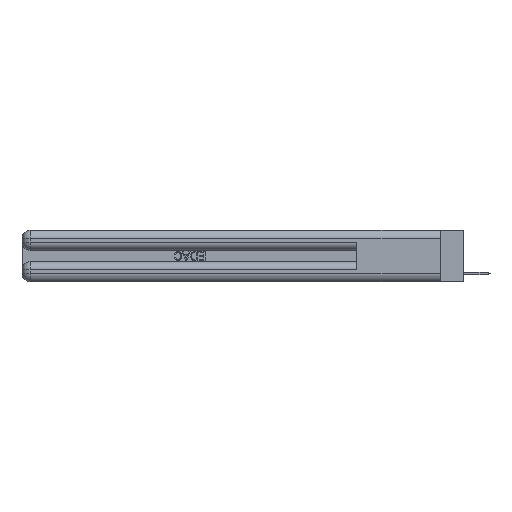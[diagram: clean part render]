
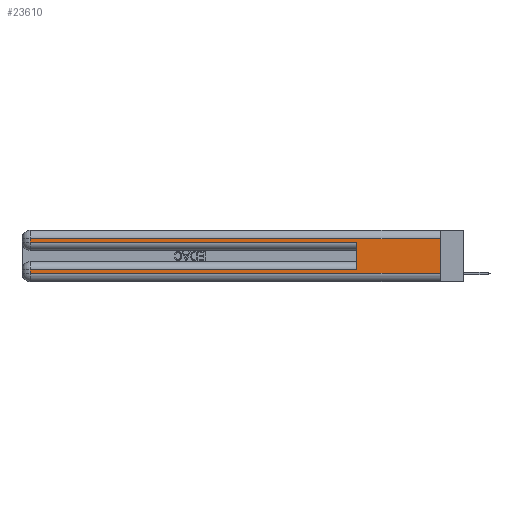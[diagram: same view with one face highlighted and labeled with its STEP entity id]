
A CAD part, left-side view. The second image highlights one B-rep face of the part: STEP entity #23610.
In plain terms, the highlighted planar face has unit normal (-1, 0, 0).
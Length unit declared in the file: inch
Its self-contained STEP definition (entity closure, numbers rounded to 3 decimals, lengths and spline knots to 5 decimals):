
#641 = CARTESIAN_POINT ( 'NONE',  ( 0., 2.94, 0.06 ) ) ;
#1298 = DIRECTION ( 'NONE',  ( 0., 1., 0. ) ) ;
#1534 = ORIENTED_EDGE ( 'NONE', *, *, #5036, .F. ) ;
#1931 = VERTEX_POINT ( 'NONE', #29692 ) ;
#2339 = VERTEX_POINT ( 'NONE', #19806 ) ;
#2497 = VERTEX_POINT ( 'NONE', #4908 ) ;
#2538 = DIRECTION ( 'NONE',  ( 0., 0., -1. ) ) ;
#2982 = DIRECTION ( 'NONE',  ( 0., 0., 1. ) ) ;
#3294 = ORIENTED_EDGE ( 'NONE', *, *, #14458, .T. ) ;
#3583 = DIRECTION ( 'NONE',  ( 0., 0., -1. ) ) ;
#4908 = CARTESIAN_POINT ( 'NONE',  ( 0., 2.94, 0.085 ) ) ;
#4956 = CARTESIAN_POINT ( 'NONE',  ( 0., 0.6, 0.145 ) ) ;
#5036 = EDGE_CURVE ( 'NONE', #18062, #2339, #28475, .T. ) ;
#5630 = VECTOR ( 'NONE', #28234, 39.37008 ) ;
#5827 = EDGE_CURVE ( 'NONE', #1931, #2339, #6057, .T. ) ;
#6057 = LINE ( 'NONE', #8047, #24144 ) ;
#6139 = LINE ( 'NONE', #10268, #23986 ) ;
#6505 = ORIENTED_EDGE ( 'NONE', *, *, #22108, .T. ) ;
#6848 = VECTOR ( 'NONE', #14466, 39.37008 ) ;
#7990 = EDGE_CURVE ( 'NONE', #18062, #2497, #6139, .T. ) ;
#8047 = CARTESIAN_POINT ( 'NONE',  ( 0., 0., 0.285 ) ) ;
#8107 = CARTESIAN_POINT ( 'NONE',  ( 0., 0., 0.06 ) ) ;
#8311 = EDGE_LOOP ( 'NONE', ( #23477, #3294, #29740, #26399, #1534, #8795, #27456, #6505 ) ) ;
#8795 = ORIENTED_EDGE ( 'NONE', *, *, #7990, .T. ) ;
#8894 = EDGE_CURVE ( 'NONE', #2497, #29119, #9076, .T. ) ;
#9076 = LINE ( 'NONE', #13944, #23434 ) ;
#9329 = CARTESIAN_POINT ( 'NONE',  ( 0., 0., 0.37 ) ) ;
#9369 = CARTESIAN_POINT ( 'NONE',  ( 0., 2.94, 0.31 ) ) ;
#10268 = CARTESIAN_POINT ( 'NONE',  ( 0., 0., 0.085 ) ) ;
#10375 = AXIS2_PLACEMENT_3D ( 'NONE', #9329, #19033, #16766 ) ;
#12205 = PLANE ( 'NONE',  #10375 ) ;
#12231 = EDGE_CURVE ( 'NONE', #15840, #27626, #17131, .T. ) ;
#13672 = CARTESIAN_POINT ( 'NONE',  ( 0., 0., 0.31 ) ) ;
#13944 = CARTESIAN_POINT ( 'NONE',  ( 0., 2.94, 0.37 ) ) ;
#14301 = LINE ( 'NONE', #18998, #5630 ) ;
#14458 = EDGE_CURVE ( 'NONE', #15840, #24329, #14301, .T. ) ;
#14466 = DIRECTION ( 'NONE',  ( 0., 0., -1. ) ) ;
#14811 = DIRECTION ( 'NONE',  ( 0., -1., 0. ) ) ;
#15018 = VECTOR ( 'NONE', #3583, 39.37008 ) ;
#15840 = VERTEX_POINT ( 'NONE', #13672 ) ;
#16766 = DIRECTION ( 'NONE',  ( 0., 0., -1. ) ) ;
#16896 = LINE ( 'NONE', #26425, #6848 ) ;
#17131 = LINE ( 'NONE', #17574, #15018 ) ;
#17574 = CARTESIAN_POINT ( 'NONE',  ( 0., 0., 0.37 ) ) ;
#17592 = CARTESIAN_POINT ( 'NONE',  ( 0., 0.6, 0.085 ) ) ;
#18062 = VERTEX_POINT ( 'NONE', #17592 ) ;
#18561 = VECTOR ( 'NONE', #14811, 39.37008 ) ;
#18998 = CARTESIAN_POINT ( 'NONE',  ( 0., 0., 0.31 ) ) ;
#19033 = DIRECTION ( 'NONE',  ( 1., 0., 0. ) ) ;
#19208 = EDGE_CURVE ( 'NONE', #24329, #1931, #16896, .T. ) ;
#19806 = CARTESIAN_POINT ( 'NONE',  ( 0., 0.6, 0.285 ) ) ;
#22108 = EDGE_CURVE ( 'NONE', #29119, #27626, #22216, .T. ) ;
#22216 = LINE ( 'NONE', #8107, #18561 ) ;
#22631 = VECTOR ( 'NONE', #2982, 39.37008 ) ;
#23434 = VECTOR ( 'NONE', #2538, 39.37008 ) ;
#23477 = ORIENTED_EDGE ( 'NONE', *, *, #12231, .F. ) ;
#23610 = ADVANCED_FACE ( 'NONE', ( #23717 ), #12205, .F. ) ;
#23717 = FACE_OUTER_BOUND ( 'NONE', #8311, .T. ) ;
#23986 = VECTOR ( 'NONE', #1298, 39.37008 ) ;
#24144 = VECTOR ( 'NONE', #24579, 39.37008 ) ;
#24329 = VERTEX_POINT ( 'NONE', #9369 ) ;
#24579 = DIRECTION ( 'NONE',  ( 0., -1., 0. ) ) ;
#25438 = CARTESIAN_POINT ( 'NONE',  ( 0., 0., 0.06 ) ) ;
#26399 = ORIENTED_EDGE ( 'NONE', *, *, #5827, .T. ) ;
#26425 = CARTESIAN_POINT ( 'NONE',  ( 0., 2.94, 0.37 ) ) ;
#27456 = ORIENTED_EDGE ( 'NONE', *, *, #8894, .T. ) ;
#27626 = VERTEX_POINT ( 'NONE', #25438 ) ;
#28234 = DIRECTION ( 'NONE',  ( 0., 1., 0. ) ) ;
#28475 = LINE ( 'NONE', #4956, #22631 ) ;
#29119 = VERTEX_POINT ( 'NONE', #641 ) ;
#29692 = CARTESIAN_POINT ( 'NONE',  ( 0., 2.94, 0.285 ) ) ;
#29740 = ORIENTED_EDGE ( 'NONE', *, *, #19208, .T. ) ;
